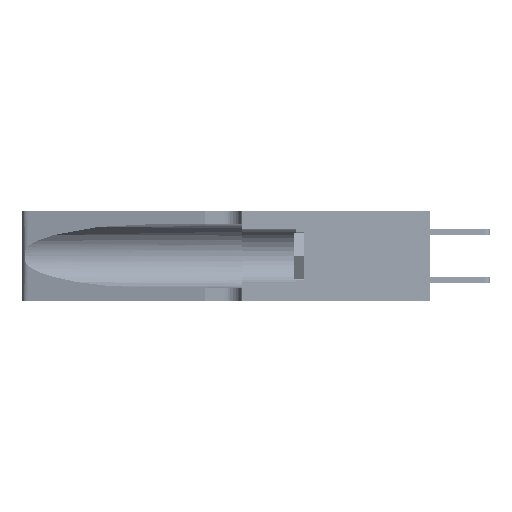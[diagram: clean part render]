
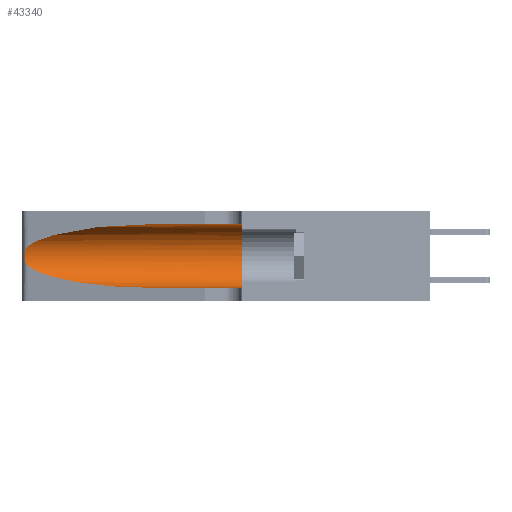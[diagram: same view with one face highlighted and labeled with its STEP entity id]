
A CAD part, left-side view. The second image highlights one B-rep face of the part: STEP entity #43340.
In plain terms, the highlighted cylindrical face has radius 3.308 mm (diameter 6.617 mm), a partial arc.
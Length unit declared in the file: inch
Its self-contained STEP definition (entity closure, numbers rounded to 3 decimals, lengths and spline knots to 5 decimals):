
#157 = CARTESIAN_POINT ( 'NONE',  ( 0.1305, 0.72297, 0.31525 ) ) ;
#464 = CARTESIAN_POINT ( 'NONE',  ( 0.25487, 1.22718, 0.14631 ) ) ;
#785 = CARTESIAN_POINT ( 'NONE',  ( 0.26075, 1.23896, 0.19203 ) ) ;
#2447 = ORIENTED_EDGE ( 'NONE', *, *, #33175, .T. ) ;
#3294 = VERTEX_POINT ( 'NONE', #14061 ) ;
#3366 = B_SPLINE_CURVE_WITH_KNOTS ( 'NONE', 3,
 ( #11388, #15227, #21945, #11074, #39849, #32270, #785, #14774, #35987, #32583, #35669, #39383, #25495, #464 ),
 .UNSPECIFIED., .F., .F.,
 ( 4, 2, 2, 2, 2, 2, 4 ),
 ( 0., 0.00027, 0.00053, 0.00107, 0.0016, 0.00187, 0.00214 ),
 .UNSPECIFIED. ) ;
#4133 = CARTESIAN_POINT ( 'NONE',  ( 0.2373, 1.15595, 0.08982 ) ) ;
#4748 = VERTEX_POINT ( 'NONE', #25968 ) ;
#5173 = AXIS2_PLACEMENT_3D ( 'NONE', #12365, #12208, #22919 ) ;
#6861 = ORIENTED_EDGE ( 'NONE', *, *, #45560, .T. ) ;
#8522 = CYLINDRICAL_SURFACE ( 'NONE', #5173, 0.13025 ) ;
#10027 = CARTESIAN_POINT ( 'NONE',  ( 0.25487, 1.22718, 0.22369 ) ) ;
#11074 = CARTESIAN_POINT ( 'NONE',  ( 0.25787, 1.23484, 0.2124 ) ) ;
#11384 = CARTESIAN_POINT ( 'NONE',  ( 0.25487, 1.22718, 0.14631 ) ) ;
#11388 = CARTESIAN_POINT ( 'NONE',  ( 0.25487, 1.22718, 0.22369 ) ) ;
#11622 = ORIENTED_EDGE ( 'NONE', *, *, #12630, .F. ) ;
#11653 = DIRECTION ( 'NONE',  ( 0., -1., 0. ) ) ;
#12208 = DIRECTION ( 'NONE',  ( 0., -1., 0. ) ) ;
#12365 = CARTESIAN_POINT ( 'NONE',  ( 0.1305, 1.61858, 0.185 ) ) ;
#12630 = EDGE_CURVE ( 'NONE', #4748, #27126, #30217, .T. ) ;
#14016 = CARTESIAN_POINT ( 'NONE',  ( 0.2373, 1.15595, 0.28018 ) ) ;
#14061 = CARTESIAN_POINT ( 'NONE',  ( 0.1305, 0.35, 0.05475 ) ) ;
#14622 = CARTESIAN_POINT ( 'NONE',  ( 0.18966, 0.96281, 0.05475 ) ) ;
#14774 = CARTESIAN_POINT ( 'NONE',  ( 0.26075, 1.23896, 0.178 ) ) ;
#15227 = CARTESIAN_POINT ( 'NONE',  ( 0.25555, 1.22994, 0.2215 ) ) ;
#16395 = EDGE_CURVE ( 'NONE', #26188, #25197, #3366, .T. ) ;
#16597 = DIRECTION ( 'NONE',  ( 0., -1., 0. ) ) ;
#16750 = CARTESIAN_POINT ( 'NONE',  ( 0.1305, 1.61858, 0.05475 ) ) ;
#18113 = AXIS2_PLACEMENT_3D ( 'NONE', #41265, #27506, #27208 ) ;
#19729 = VERTEX_POINT ( 'NONE', #20766 ) ;
#20766 = CARTESIAN_POINT ( 'NONE',  ( 0.1305, 0.72297, 0.05475 ) ) ;
#21091 =( BOUNDED_CURVE ( )  B_SPLINE_CURVE ( 3, ( #157, #45254, #14016, #10027 ),
 .UNSPECIFIED., .F., .F. ) 
 B_SPLINE_CURVE_WITH_KNOTS ( ( 4, 4 ),
 ( 1.5708, 2.84003 ),
 .UNSPECIFIED. ) 
 CURVE ( )  GEOMETRIC_REPRESENTATION_ITEM ( )  RATIONAL_B_SPLINE_CURVE ( ( 1., 0.87, 0.87, 1. ) ) 
 REPRESENTATION_ITEM ( '' )  );
#21607 = CARTESIAN_POINT ( 'NONE',  ( 0.1305, 1.61858, 0.31525 ) ) ;
#21945 = CARTESIAN_POINT ( 'NONE',  ( 0.25639, 1.23184, 0.21858 ) ) ;
#22919 = DIRECTION ( 'NONE',  ( 0., 0., -1. ) ) ;
#23881 = EDGE_CURVE ( 'NONE', #27126, #3294, #38186, .T. ) ;
#25197 = VERTEX_POINT ( 'NONE', #27872 ) ;
#25495 = CARTESIAN_POINT ( 'NONE',  ( 0.25555, 1.22993, 0.14849 ) ) ;
#25968 = CARTESIAN_POINT ( 'NONE',  ( 0.1305, 0.72297, 0.31525 ) ) ;
#26188 = VERTEX_POINT ( 'NONE', #27458 ) ;
#27126 = VERTEX_POINT ( 'NONE', #40074 ) ;
#27208 = DIRECTION ( 'NONE',  ( 0., 0., 1. ) ) ;
#27248 = LINE ( 'NONE', #16750, #34994 ) ;
#27458 = CARTESIAN_POINT ( 'NONE',  ( 0.25487, 1.22718, 0.22369 ) ) ;
#27506 = DIRECTION ( 'NONE',  ( 0., 1., 0. ) ) ;
#27872 = CARTESIAN_POINT ( 'NONE',  ( 0.25487, 1.22718, 0.14631 ) ) ;
#28737 = CARTESIAN_POINT ( 'NONE',  ( 0.1305, 0.72297, 0.05475 ) ) ;
#29314 =( BOUNDED_CURVE ( )  B_SPLINE_CURVE ( 3, ( #11384, #4133, #14622, #28737 ),
 .UNSPECIFIED., .F., .F. ) 
 B_SPLINE_CURVE_WITH_KNOTS ( ( 4, 4 ),
 ( 3.44316, 4.71239 ),
 .UNSPECIFIED. ) 
 CURVE ( )  GEOMETRIC_REPRESENTATION_ITEM ( )  RATIONAL_B_SPLINE_CURVE ( ( 1., 0.87, 0.87, 1. ) ) 
 REPRESENTATION_ITEM ( '' )  );
#30217 = LINE ( 'NONE', #21607, #32427 ) ;
#30698 = ORIENTED_EDGE ( 'NONE', *, *, #16395, .T. ) ;
#32270 = CARTESIAN_POINT ( 'NONE',  ( 0.26018, 1.23835, 0.19895 ) ) ;
#32427 = VECTOR ( 'NONE', #11653, 39.37008 ) ;
#32583 = CARTESIAN_POINT ( 'NONE',  ( 0.25856, 1.23593, 0.16098 ) ) ;
#33175 = EDGE_CURVE ( 'NONE', #25197, #19729, #29314, .T. ) ;
#33845 = EDGE_LOOP ( 'NONE', ( #44172, #30698, #2447, #6861, #41471, #11622 ) ) ;
#34994 = VECTOR ( 'NONE', #16597, 39.37008 ) ;
#35669 = CARTESIAN_POINT ( 'NONE',  ( 0.25789, 1.23486, 0.15765 ) ) ;
#35987 = CARTESIAN_POINT ( 'NONE',  ( 0.26017, 1.23833, 0.17102 ) ) ;
#38186 = CIRCLE ( 'NONE', #18113, 0.13025 ) ;
#39325 = FACE_OUTER_BOUND ( 'NONE', #33845, .T. ) ;
#39383 = CARTESIAN_POINT ( 'NONE',  ( 0.25639, 1.23186, 0.15144 ) ) ;
#39849 = CARTESIAN_POINT ( 'NONE',  ( 0.25854, 1.2359, 0.20912 ) ) ;
#40074 = CARTESIAN_POINT ( 'NONE',  ( 0.1305, 0.35, 0.31525 ) ) ;
#41265 = CARTESIAN_POINT ( 'NONE',  ( 0.1305, 0.35, 0.185 ) ) ;
#41471 = ORIENTED_EDGE ( 'NONE', *, *, #23881, .F. ) ;
#43340 = ADVANCED_FACE ( 'NONE', ( #39325 ), #8522, .F. ) ;
#43730 = EDGE_CURVE ( 'NONE', #4748, #26188, #21091, .T. ) ;
#44172 = ORIENTED_EDGE ( 'NONE', *, *, #43730, .T. ) ;
#45254 = CARTESIAN_POINT ( 'NONE',  ( 0.18966, 0.96281, 0.31525 ) ) ;
#45560 = EDGE_CURVE ( 'NONE', #19729, #3294, #27248, .T. ) ;
